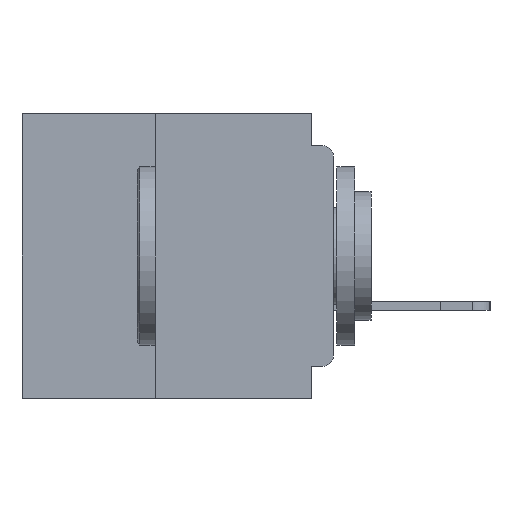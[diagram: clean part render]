
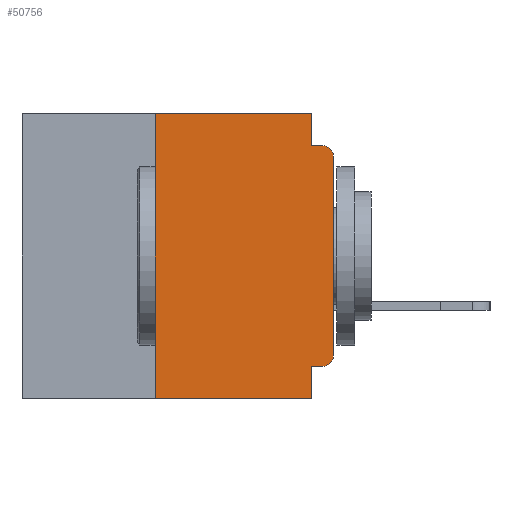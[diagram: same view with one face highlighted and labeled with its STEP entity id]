
A CAD part, left-side view. The second image highlights one B-rep face of the part: STEP entity #50756.
In plain terms, the highlighted planar face has unit normal (-1, 0, 0).
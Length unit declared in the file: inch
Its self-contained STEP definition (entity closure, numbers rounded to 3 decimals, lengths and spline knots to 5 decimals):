
#1822 = AXIS2_PLACEMENT_3D ( 'NONE', #37450, #11626, #41789 ) ;
#3966 = EDGE_LOOP ( 'NONE', ( #36027, #51650, #40124, #53574, #44152, #42090, #20527, #47570, #47223, #46689 ) ) ;
#4421 = VERTEX_POINT ( 'NONE', #34156 ) ;
#5594 = AXIS2_PLACEMENT_3D ( 'NONE', #14170, #44359, #18535 ) ;
#6171 = VERTEX_POINT ( 'NONE', #10244 ) ;
#7489 = CARTESIAN_POINT ( 'NONE',  ( 0., 0., 0. ) ) ;
#8115 = DIRECTION ( 'NONE',  ( 0., 0., -1. ) ) ;
#8116 = VECTOR ( 'NONE', #41953, 39.37008 ) ;
#8768 = VECTOR ( 'NONE', #17436, 39.37008 ) ;
#9176 = CARTESIAN_POINT ( 'NONE',  ( 0., 0.015, -0.045 ) ) ;
#9306 = EDGE_CURVE ( 'NONE', #36943, #28187, #43200, .T. ) ;
#9590 = EDGE_CURVE ( 'NONE', #49174, #4421, #49914, .T. ) ;
#9861 = PLANE ( 'NONE',  #5594 ) ;
#10244 = CARTESIAN_POINT ( 'NONE',  ( 0., 0.25, -0.4 ) ) ;
#10936 = FACE_OUTER_BOUND ( 'NONE', #3966, .T. ) ;
#11626 = DIRECTION ( 'NONE',  ( -1., 0., 0. ) ) ;
#14056 = CIRCLE ( 'NONE', #1822, 0.015 ) ;
#14170 = CARTESIAN_POINT ( 'NONE',  ( 0., 0.437, 0. ) ) ;
#14948 = VERTEX_POINT ( 'NONE', #43343 ) ;
#15166 = CARTESIAN_POINT ( 'NONE',  ( 0., 0.031, -0.045 ) ) ;
#17436 = DIRECTION ( 'NONE',  ( 0., -1., 0. ) ) ;
#17994 = VERTEX_POINT ( 'NONE', #15166 ) ;
#18535 = DIRECTION ( 'NONE',  ( 0., 0., -1. ) ) ;
#18935 = VERTEX_POINT ( 'NONE', #26992 ) ;
#19655 = DIRECTION ( 'NONE',  ( -1., 0., 0. ) ) ;
#20207 = LINE ( 'NONE', #21782, #8768 ) ;
#20302 = VECTOR ( 'NONE', #36715, 39.37008 ) ;
#20527 = ORIENTED_EDGE ( 'NONE', *, *, #37991, .T. ) ;
#21782 = CARTESIAN_POINT ( 'NONE',  ( 0., 0.437, -0.4 ) ) ;
#22289 = LINE ( 'NONE', #7489, #8116 ) ;
#22331 = VERTEX_POINT ( 'NONE', #9176 ) ;
#22721 = LINE ( 'NONE', #25025, #45633 ) ;
#24354 = LINE ( 'NONE', #39509, #48619 ) ;
#24902 = EDGE_CURVE ( 'NONE', #47833, #49174, #24354, .T. ) ;
#25025 = CARTESIAN_POINT ( 'NONE',  ( 0., 0.25, -0.4 ) ) ;
#26992 = CARTESIAN_POINT ( 'NONE',  ( 0., 0., -0.34 ) ) ;
#28187 = VERTEX_POINT ( 'NONE', #37782 ) ;
#31400 = CARTESIAN_POINT ( 'NONE',  ( 0., 0.015, -0.355 ) ) ;
#31763 = VECTOR ( 'NONE', #40368, 39.37008 ) ;
#32392 = CARTESIAN_POINT ( 'NONE',  ( 0., 0., -0.045 ) ) ;
#32500 = LINE ( 'NONE', #35221, #52695 ) ;
#33877 = CARTESIAN_POINT ( 'NONE',  ( 0., 0.25, 0. ) ) ;
#34156 = CARTESIAN_POINT ( 'NONE',  ( 0., 0.031, -0.4 ) ) ;
#35221 = CARTESIAN_POINT ( 'NONE',  ( 0., 0.031, 0. ) ) ;
#35609 = EDGE_CURVE ( 'NONE', #14948, #22331, #47510, .T. ) ;
#36027 = ORIENTED_EDGE ( 'NONE', *, *, #37785, .T. ) ;
#36532 = EDGE_CURVE ( 'NONE', #28187, #17994, #32500, .T. ) ;
#36715 = DIRECTION ( 'NONE',  ( 0., -1., 0. ) ) ;
#36726 = EDGE_CURVE ( 'NONE', #17994, #22331, #54683, .T. ) ;
#36943 = VERTEX_POINT ( 'NONE', #33877 ) ;
#37450 = CARTESIAN_POINT ( 'NONE',  ( 0., 0.015, -0.34 ) ) ;
#37782 = CARTESIAN_POINT ( 'NONE',  ( 0., 0.031, 0. ) ) ;
#37785 = EDGE_CURVE ( 'NONE', #18935, #14948, #22289, .T. ) ;
#37991 = EDGE_CURVE ( 'NONE', #6171, #4421, #20207, .T. ) ;
#38060 = CARTESIAN_POINT ( 'NONE',  ( 0., 0.031, -0.4 ) ) ;
#38459 = VECTOR ( 'NONE', #8115, 39.37008 ) ;
#38561 = DIRECTION ( 'NONE',  ( 0., 1., 0. ) ) ;
#39509 = CARTESIAN_POINT ( 'NONE',  ( 0., 0., -0.355 ) ) ;
#40124 = ORIENTED_EDGE ( 'NONE', *, *, #36726, .F. ) ;
#40368 = DIRECTION ( 'NONE',  ( 0., -1., 0. ) ) ;
#41772 = AXIS2_PLACEMENT_3D ( 'NONE', #45486, #19655, #49815 ) ;
#41789 = DIRECTION ( 'NONE',  ( 0., 0., -1. ) ) ;
#41953 = DIRECTION ( 'NONE',  ( 0., 0., 1. ) ) ;
#42090 = ORIENTED_EDGE ( 'NONE', *, *, #54046, .F. ) ;
#43200 = LINE ( 'NONE', #53168, #31763 ) ;
#43343 = CARTESIAN_POINT ( 'NONE',  ( 0., 0., -0.06 ) ) ;
#44152 = ORIENTED_EDGE ( 'NONE', *, *, #9306, .F. ) ;
#44359 = DIRECTION ( 'NONE',  ( 1., 0., 0. ) ) ;
#45486 = CARTESIAN_POINT ( 'NONE',  ( 0., 0.015, -0.06 ) ) ;
#45633 = VECTOR ( 'NONE', #50812, 39.37008 ) ;
#46689 = ORIENTED_EDGE ( 'NONE', *, *, #55738, .T. ) ;
#47223 = ORIENTED_EDGE ( 'NONE', *, *, #24902, .F. ) ;
#47510 = CIRCLE ( 'NONE', #41772, 0.015 ) ;
#47570 = ORIENTED_EDGE ( 'NONE', *, *, #9590, .F. ) ;
#47833 = VERTEX_POINT ( 'NONE', #31400 ) ;
#48619 = VECTOR ( 'NONE', #38561, 39.37008 ) ;
#49174 = VERTEX_POINT ( 'NONE', #54862 ) ;
#49815 = DIRECTION ( 'NONE',  ( 0., 0., -1. ) ) ;
#49914 = LINE ( 'NONE', #38060, #38459 ) ;
#50756 = ADVANCED_FACE ( 'NONE', ( #10936 ), #9861, .F. ) ;
#50812 = DIRECTION ( 'NONE',  ( 0., 0., 1. ) ) ;
#51650 = ORIENTED_EDGE ( 'NONE', *, *, #35609, .T. ) ;
#52374 = DIRECTION ( 'NONE',  ( 0., 0., -1. ) ) ;
#52695 = VECTOR ( 'NONE', #52374, 39.37008 ) ;
#53168 = CARTESIAN_POINT ( 'NONE',  ( 0., 0.437, 0. ) ) ;
#53574 = ORIENTED_EDGE ( 'NONE', *, *, #36532, .F. ) ;
#54046 = EDGE_CURVE ( 'NONE', #6171, #36943, #22721, .T. ) ;
#54683 = LINE ( 'NONE', #32392, #20302 ) ;
#54862 = CARTESIAN_POINT ( 'NONE',  ( 0., 0.031, -0.355 ) ) ;
#55738 = EDGE_CURVE ( 'NONE', #47833, #18935, #14056, .T. ) ;
